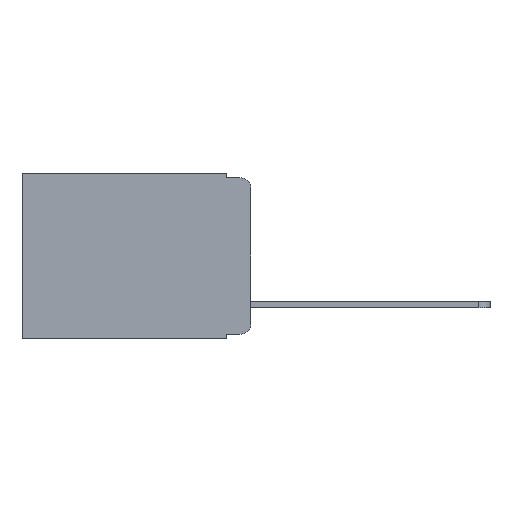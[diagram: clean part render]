
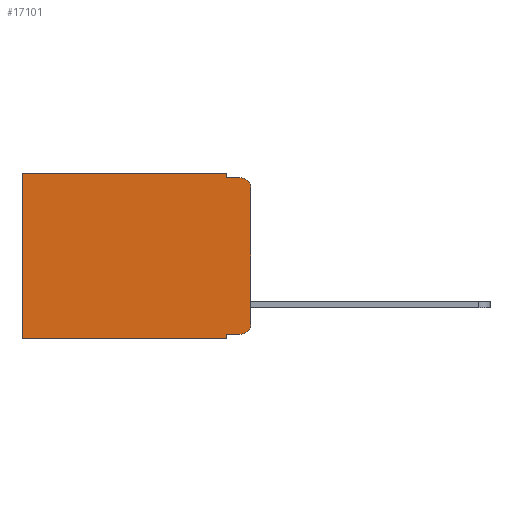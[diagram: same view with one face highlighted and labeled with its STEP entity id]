
A CAD part, left-side view. The second image highlights one B-rep face of the part: STEP entity #17101.
In plain terms, the highlighted planar face has unit normal (-1, 0, 0).
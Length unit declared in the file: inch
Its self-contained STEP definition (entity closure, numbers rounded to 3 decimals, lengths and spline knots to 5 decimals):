
#29 = ORIENTED_EDGE ( 'NONE', *, *, #1231, .F. ) ;
#239 = DIRECTION ( 'NONE',  ( 0., 1., 0. ) ) ;
#300 = DIRECTION ( 'NONE',  ( 0., 1., 0. ) ) ;
#527 = LINE ( 'NONE', #11049, #19337 ) ;
#825 = VERTEX_POINT ( 'NONE', #6260 ) ;
#1090 = LINE ( 'NONE', #12025, #7251 ) ;
#1231 = EDGE_CURVE ( 'NONE', #22391, #21112, #14798, .T. ) ;
#2437 = EDGE_CURVE ( 'NONE', #11790, #10080, #5972, .T. ) ;
#2586 = AXIS2_PLACEMENT_3D ( 'NONE', #5816, #6041, #18515 ) ;
#2669 = VECTOR ( 'NONE', #11917, 39.37008 ) ;
#2786 = VECTOR ( 'NONE', #239, 39.37008 ) ;
#2829 = CARTESIAN_POINT ( 'NONE',  ( 0.298, 0.473, 0. ) ) ;
#3000 = EDGE_CURVE ( 'NONE', #23242, #8439, #8746, .T. ) ;
#3372 = AXIS2_PLACEMENT_3D ( 'NONE', #12500, #7274, #19749 ) ;
#3899 = ORIENTED_EDGE ( 'NONE', *, *, #13647, .F. ) ;
#4399 = VECTOR ( 'NONE', #8048, 39.37008 ) ;
#4793 = FACE_OUTER_BOUND ( 'NONE', #10662, .T. ) ;
#5304 = EDGE_CURVE ( 'NONE', #17173, #8439, #9435, .T. ) ;
#5388 = PLANE ( 'NONE',  #3372 ) ;
#5429 = CARTESIAN_POINT ( 'NONE',  ( 0.298, 0., -0.313 ) ) ;
#5531 = CARTESIAN_POINT ( 'NONE',  ( 0.298, 0.473, -0.343 ) ) ;
#5816 = CARTESIAN_POINT ( 'NONE',  ( 0.298, 0.02, -0.313 ) ) ;
#5900 = VERTEX_POINT ( 'NONE', #14915 ) ;
#5972 = CIRCLE ( 'NONE', #2586, 0.02 ) ;
#6041 = DIRECTION ( 'NONE',  ( -1., 0., 0. ) ) ;
#6260 = CARTESIAN_POINT ( 'NONE',  ( 0.298, 0.051, 0. ) ) ;
#6337 = AXIS2_PLACEMENT_3D ( 'NONE', #9268, #16190, #7440 ) ;
#6440 = ORIENTED_EDGE ( 'NONE', *, *, #12771, .T. ) ;
#6784 = VECTOR ( 'NONE', #300, 39.37008 ) ;
#7251 = VECTOR ( 'NONE', #8382, 39.37008 ) ;
#7274 = DIRECTION ( 'NONE',  ( 1., 0., 0. ) ) ;
#7440 = DIRECTION ( 'NONE',  ( 0., 0., -1. ) ) ;
#8048 = DIRECTION ( 'NONE',  ( 0., 0., -1. ) ) ;
#8382 = DIRECTION ( 'NONE',  ( 0., 0., -1. ) ) ;
#8439 = VERTEX_POINT ( 'NONE', #5531 ) ;
#8746 = LINE ( 'NONE', #19982, #6784 ) ;
#8814 = CARTESIAN_POINT ( 'NONE',  ( 0.298, 0.02, -0.333 ) ) ;
#9095 = CARTESIAN_POINT ( 'NONE',  ( 0.298, 0., 0. ) ) ;
#9268 = CARTESIAN_POINT ( 'NONE',  ( 0.298, 0.02, -0.03 ) ) ;
#9435 = LINE ( 'NONE', #2829, #2669 ) ;
#9720 = VECTOR ( 'NONE', #19661, 39.37008 ) ;
#10080 = VERTEX_POINT ( 'NONE', #5429 ) ;
#10662 = EDGE_LOOP ( 'NONE', ( #13526, #21762, #29, #14511, #18827, #23035, #19602, #3899, #6440, #12060 ) ) ;
#10785 = EDGE_CURVE ( 'NONE', #5900, #21112, #18682, .T. ) ;
#10910 = DIRECTION ( 'NONE',  ( 0., 0., -1. ) ) ;
#11049 = CARTESIAN_POINT ( 'NONE',  ( 0.298, 0.051, -0.333 ) ) ;
#11790 = VERTEX_POINT ( 'NONE', #8814 ) ;
#11917 = DIRECTION ( 'NONE',  ( 0., 0., -1. ) ) ;
#12025 = CARTESIAN_POINT ( 'NONE',  ( 0.298, 0.051, 0. ) ) ;
#12060 = ORIENTED_EDGE ( 'NONE', *, *, #2437, .T. ) ;
#12314 = LINE ( 'NONE', #20504, #4399 ) ;
#12500 = CARTESIAN_POINT ( 'NONE',  ( 0.298, 0., 0. ) ) ;
#12771 = EDGE_CURVE ( 'NONE', #14831, #11790, #527, .T. ) ;
#12859 = CARTESIAN_POINT ( 'NONE',  ( 0.298, 0.051, -0.01 ) ) ;
#12905 = CARTESIAN_POINT ( 'NONE',  ( 0.298, 0., 0. ) ) ;
#13424 = CARTESIAN_POINT ( 'NONE',  ( 0.298, 0.051, -0.343 ) ) ;
#13526 = ORIENTED_EDGE ( 'NONE', *, *, #13891, .F. ) ;
#13647 = EDGE_CURVE ( 'NONE', #14831, #23242, #1090, .T. ) ;
#13891 = EDGE_CURVE ( 'NONE', #5900, #10080, #19315, .T. ) ;
#14170 = EDGE_CURVE ( 'NONE', #825, #22391, #12314, .T. ) ;
#14511 = ORIENTED_EDGE ( 'NONE', *, *, #14170, .F. ) ;
#14689 = CARTESIAN_POINT ( 'NONE',  ( 0.298, 0.473, 0. ) ) ;
#14798 = LINE ( 'NONE', #16088, #9720 ) ;
#14831 = VERTEX_POINT ( 'NONE', #22272 ) ;
#14847 = VECTOR ( 'NONE', #10910, 39.37008 ) ;
#14915 = CARTESIAN_POINT ( 'NONE',  ( 0.298, 0., -0.03 ) ) ;
#16088 = CARTESIAN_POINT ( 'NONE',  ( 0.298, 0.051, -0.01 ) ) ;
#16190 = DIRECTION ( 'NONE',  ( -1., 0., 0. ) ) ;
#16340 = CARTESIAN_POINT ( 'NONE',  ( 0.298, 0.02, -0.01 ) ) ;
#17101 = ADVANCED_FACE ( 'NONE', ( #4793 ), #5388, .F. ) ;
#17173 = VERTEX_POINT ( 'NONE', #14689 ) ;
#18515 = DIRECTION ( 'NONE',  ( 0., 0., -1. ) ) ;
#18682 = CIRCLE ( 'NONE', #6337, 0.02 ) ;
#18827 = ORIENTED_EDGE ( 'NONE', *, *, #23048, .T. ) ;
#19315 = LINE ( 'NONE', #9095, #14847 ) ;
#19337 = VECTOR ( 'NONE', #21498, 39.37008 ) ;
#19602 = ORIENTED_EDGE ( 'NONE', *, *, #3000, .F. ) ;
#19661 = DIRECTION ( 'NONE',  ( 0., -1., 0. ) ) ;
#19749 = DIRECTION ( 'NONE',  ( 0., 0., -1. ) ) ;
#19982 = CARTESIAN_POINT ( 'NONE',  ( 0.298, 0., -0.343 ) ) ;
#20504 = CARTESIAN_POINT ( 'NONE',  ( 0.298, 0.051, 0. ) ) ;
#21112 = VERTEX_POINT ( 'NONE', #16340 ) ;
#21498 = DIRECTION ( 'NONE',  ( 0., -1., 0. ) ) ;
#21600 = LINE ( 'NONE', #12905, #2786 ) ;
#21762 = ORIENTED_EDGE ( 'NONE', *, *, #10785, .T. ) ;
#22272 = CARTESIAN_POINT ( 'NONE',  ( 0.298, 0.051, -0.333 ) ) ;
#22391 = VERTEX_POINT ( 'NONE', #12859 ) ;
#23035 = ORIENTED_EDGE ( 'NONE', *, *, #5304, .T. ) ;
#23048 = EDGE_CURVE ( 'NONE', #825, #17173, #21600, .T. ) ;
#23242 = VERTEX_POINT ( 'NONE', #13424 ) ;
